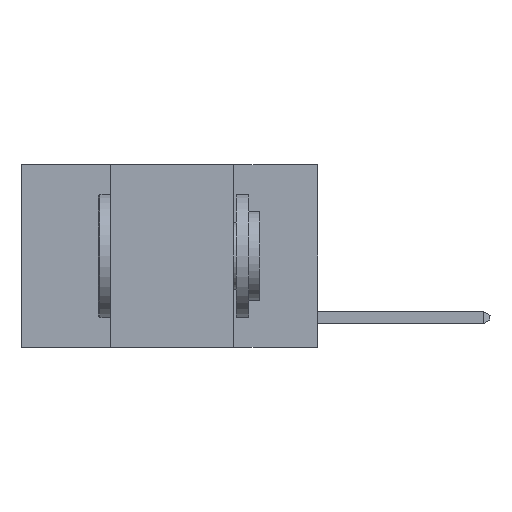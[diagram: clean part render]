
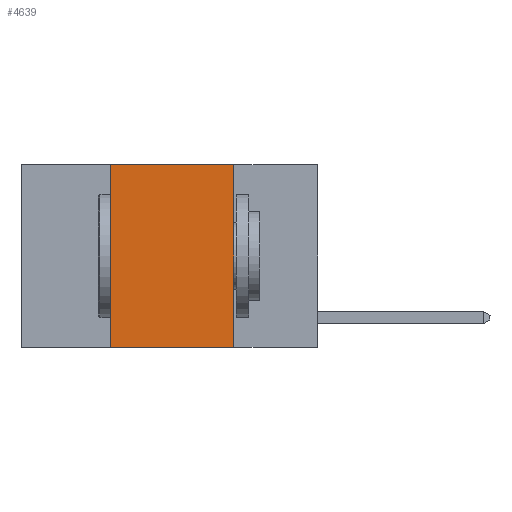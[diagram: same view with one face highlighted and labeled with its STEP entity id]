
A CAD part, left-side view. The second image highlights one B-rep face of the part: STEP entity #4639.
In plain terms, the highlighted planar face has unit normal (-1, 0, 0).
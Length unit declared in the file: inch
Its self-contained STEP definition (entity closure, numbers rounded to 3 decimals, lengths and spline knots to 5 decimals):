
#708 = CARTESIAN_POINT ( 'NONE',  ( 0., 0.6, 0. ) ) ;
#770 = PLANE ( 'NONE',  #16746 ) ;
#841 = ORIENTED_EDGE ( 'NONE', *, *, #12839, .F. ) ;
#963 = CARTESIAN_POINT ( 'NONE',  ( 0., 0.42, -0.37 ) ) ;
#1162 = LINE ( 'NONE', #4858, #16729 ) ;
#1234 = ORIENTED_EDGE ( 'NONE', *, *, #16416, .F. ) ;
#1568 = CARTESIAN_POINT ( 'NONE',  ( 0., 0.42, 0. ) ) ;
#2302 = DIRECTION ( 'NONE',  ( 0., 0., -1. ) ) ;
#3368 = VECTOR ( 'NONE', #18902, 39.37008 ) ;
#3849 = CARTESIAN_POINT ( 'NONE',  ( 0., 0.17, 0. ) ) ;
#3969 = VECTOR ( 'NONE', #17329, 39.37008 ) ;
#4639 = ADVANCED_FACE ( 'NONE', ( #19269 ), #770, .F. ) ;
#4858 = CARTESIAN_POINT ( 'NONE',  ( 0., 0.6, -0.37 ) ) ;
#5462 = VERTEX_POINT ( 'NONE', #16154 ) ;
#6181 = LINE ( 'NONE', #9162, #10214 ) ;
#6205 = VERTEX_POINT ( 'NONE', #1568 ) ;
#7137 = EDGE_LOOP ( 'NONE', ( #1234, #8860, #841, #9301 ) ) ;
#8860 = ORIENTED_EDGE ( 'NONE', *, *, #11215, .F. ) ;
#9162 = CARTESIAN_POINT ( 'NONE',  ( 0., 0.6, 0. ) ) ;
#9301 = ORIENTED_EDGE ( 'NONE', *, *, #10835, .T. ) ;
#10041 = CARTESIAN_POINT ( 'NONE',  ( 0., 0.17, -0.37 ) ) ;
#10214 = VECTOR ( 'NONE', #16570, 39.37008 ) ;
#10495 = VERTEX_POINT ( 'NONE', #963 ) ;
#10835 = EDGE_CURVE ( 'NONE', #10495, #15503, #1162, .T. ) ;
#11215 = EDGE_CURVE ( 'NONE', #6205, #5462, #6181, .T. ) ;
#11405 = DIRECTION ( 'NONE',  ( 1., 0., 0. ) ) ;
#11420 = LINE ( 'NONE', #3849, #3368 ) ;
#11995 = LINE ( 'NONE', #15811, #3969 ) ;
#12839 = EDGE_CURVE ( 'NONE', #10495, #6205, #11995, .T. ) ;
#13909 = DIRECTION ( 'NONE',  ( 0., -1., 0. ) ) ;
#15503 = VERTEX_POINT ( 'NONE', #10041 ) ;
#15811 = CARTESIAN_POINT ( 'NONE',  ( 0., 0.42, 0. ) ) ;
#16154 = CARTESIAN_POINT ( 'NONE',  ( 0., 0.17, 0. ) ) ;
#16416 = EDGE_CURVE ( 'NONE', #5462, #15503, #11420, .T. ) ;
#16570 = DIRECTION ( 'NONE',  ( 0., -1., 0. ) ) ;
#16729 = VECTOR ( 'NONE', #13909, 39.37008 ) ;
#16746 = AXIS2_PLACEMENT_3D ( 'NONE', #708, #11405, #2302 ) ;
#17329 = DIRECTION ( 'NONE',  ( 0., 0., 1. ) ) ;
#18902 = DIRECTION ( 'NONE',  ( 0., 0., -1. ) ) ;
#19269 = FACE_OUTER_BOUND ( 'NONE', #7137, .T. ) ;
